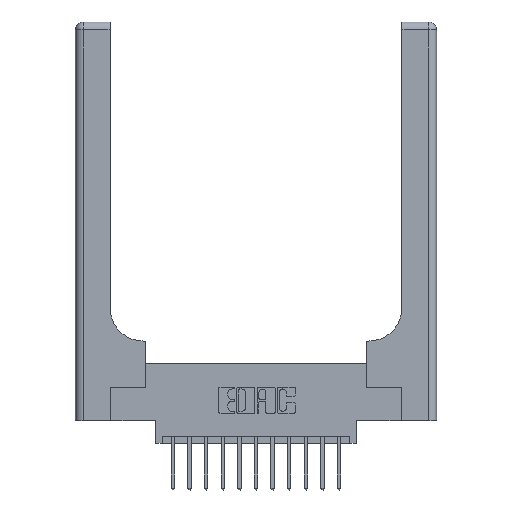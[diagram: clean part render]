
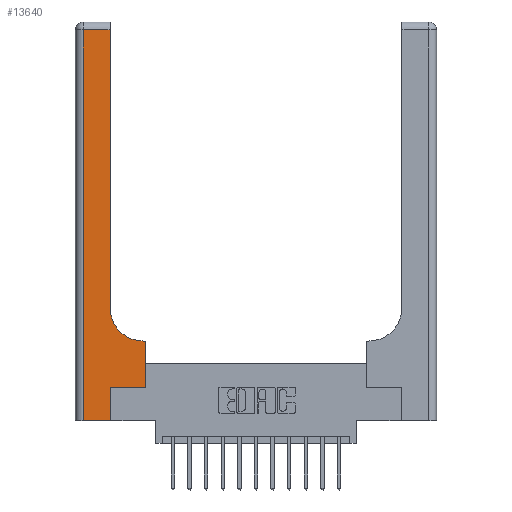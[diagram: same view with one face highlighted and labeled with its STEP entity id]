
A CAD part, top view. The second image highlights one B-rep face of the part: STEP entity #13640.
In plain terms, the highlighted planar face has unit normal (0, 0, 1).
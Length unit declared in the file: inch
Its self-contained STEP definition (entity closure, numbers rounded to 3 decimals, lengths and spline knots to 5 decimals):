
#272 = CARTESIAN_POINT ( 'NONE',  ( 0.265, 0.25, 0.37 ) ) ;
#301 = VECTOR ( 'NONE', #4578, 39.37008 ) ;
#364 = DIRECTION ( 'NONE',  ( 0., 1., 0. ) ) ;
#718 = CARTESIAN_POINT ( 'NONE',  ( 0., 0., 0.37 ) ) ;
#1066 = VECTOR ( 'NONE', #2626, 39.37008 ) ;
#1144 = CARTESIAN_POINT ( 'NONE',  ( 0.265, 0.25, 0.37 ) ) ;
#1217 = DIRECTION ( 'NONE',  ( 1., 0., 0. ) ) ;
#1365 = DIRECTION ( 'NONE',  ( 0., 0., -1. ) ) ;
#1498 = LINE ( 'NONE', #3154, #15614 ) ;
#1693 = EDGE_CURVE ( 'NONE', #6602, #12836, #7559, .T. ) ;
#1719 = CARTESIAN_POINT ( 'NONE',  ( 0., 2.94, 0.37 ) ) ;
#1975 = VERTEX_POINT ( 'NONE', #7046 ) ;
#2366 = EDGE_CURVE ( 'NONE', #8411, #1975, #9901, .T. ) ;
#2603 = ORIENTED_EDGE ( 'NONE', *, *, #16585, .T. ) ;
#2626 = DIRECTION ( 'NONE',  ( -1., 0., 0. ) ) ;
#3154 = CARTESIAN_POINT ( 'NONE',  ( 0.26, 3., 0.37 ) ) ;
#3428 = ORIENTED_EDGE ( 'NONE', *, *, #12887, .T. ) ;
#4018 = VERTEX_POINT ( 'NONE', #6866 ) ;
#4449 = LINE ( 'NONE', #7739, #1066 ) ;
#4478 = EDGE_CURVE ( 'NONE', #4018, #6602, #14662, .T. ) ;
#4578 = DIRECTION ( 'NONE',  ( 1., 0., 0. ) ) ;
#4962 = CARTESIAN_POINT ( 'NONE',  ( 0.528, 0.6, 0.37 ) ) ;
#5374 = EDGE_CURVE ( 'NONE', #12836, #7989, #5957, .T. ) ;
#5444 = CARTESIAN_POINT ( 'NONE',  ( 0.51, 0.85, 0.37 ) ) ;
#5725 = VECTOR ( 'NONE', #9416, 39.37008 ) ;
#5957 = LINE ( 'NONE', #13205, #12016 ) ;
#6065 = DIRECTION ( 'NONE',  ( 0., 1., 0. ) ) ;
#6602 = VERTEX_POINT ( 'NONE', #272 ) ;
#6757 = DIRECTION ( 'NONE',  ( 1., 0., 0. ) ) ;
#6866 = CARTESIAN_POINT ( 'NONE',  ( 0.265, 0., 0.37 ) ) ;
#7046 = CARTESIAN_POINT ( 'NONE',  ( 0.26, 0.85, 0.37 ) ) ;
#7147 = LINE ( 'NONE', #718, #301 ) ;
#7559 = LINE ( 'NONE', #1144, #10982 ) ;
#7636 = EDGE_CURVE ( 'NONE', #11572, #14128, #11759, .T. ) ;
#7713 = AXIS2_PLACEMENT_3D ( 'NONE', #9073, #1365, #10384 ) ;
#7739 = CARTESIAN_POINT ( 'NONE',  ( 0.26, 0.6, 0.37 ) ) ;
#7812 = VECTOR ( 'NONE', #6065, 39.37008 ) ;
#7989 = VERTEX_POINT ( 'NONE', #4962 ) ;
#8200 = CARTESIAN_POINT ( 'NONE',  ( 0.26, 2.94, 0.37 ) ) ;
#8296 = AXIS2_PLACEMENT_3D ( 'NONE', #5444, #14469, #6757 ) ;
#8310 = VECTOR ( 'NONE', #11907, 39.37008 ) ;
#8411 = VERTEX_POINT ( 'NONE', #8564 ) ;
#8476 = ORIENTED_EDGE ( 'NONE', *, *, #4478, .T. ) ;
#8564 = CARTESIAN_POINT ( 'NONE',  ( 0.51, 0.6, 0.37 ) ) ;
#8586 = ORIENTED_EDGE ( 'NONE', *, *, #7636, .T. ) ;
#8614 = CARTESIAN_POINT ( 'NONE',  ( 0.265, 0., 0.37 ) ) ;
#9073 = CARTESIAN_POINT ( 'NONE',  ( 0., 3., 0.37 ) ) ;
#9416 = DIRECTION ( 'NONE',  ( -1., 0., 0. ) ) ;
#9901 = CIRCLE ( 'NONE', #8296, 0.25 ) ;
#10336 = PLANE ( 'NONE',  #7713 ) ;
#10384 = DIRECTION ( 'NONE',  ( -1., 0., 0. ) ) ;
#10615 = CARTESIAN_POINT ( 'NONE',  ( 0.06, 3., 0.37 ) ) ;
#10982 = VECTOR ( 'NONE', #1217, 39.37008 ) ;
#11483 = VERTEX_POINT ( 'NONE', #8200 ) ;
#11572 = VERTEX_POINT ( 'NONE', #15028 ) ;
#11587 = EDGE_LOOP ( 'NONE', ( #2603, #16291, #8586, #3428, #8476, #13441, #15193, #12345, #12212 ) ) ;
#11759 = LINE ( 'NONE', #10615, #8310 ) ;
#11907 = DIRECTION ( 'NONE',  ( 0., -1., 0. ) ) ;
#12016 = VECTOR ( 'NONE', #364, 39.37008 ) ;
#12049 = EDGE_CURVE ( 'NONE', #11483, #11572, #15628, .T. ) ;
#12169 = DIRECTION ( 'NONE',  ( 0., 1., 0. ) ) ;
#12212 = ORIENTED_EDGE ( 'NONE', *, *, #2366, .T. ) ;
#12345 = ORIENTED_EDGE ( 'NONE', *, *, #14815, .T. ) ;
#12746 = CARTESIAN_POINT ( 'NONE',  ( 0.06, 0., 0.37 ) ) ;
#12836 = VERTEX_POINT ( 'NONE', #13487 ) ;
#12887 = EDGE_CURVE ( 'NONE', #14128, #4018, #7147, .T. ) ;
#12986 = FACE_OUTER_BOUND ( 'NONE', #11587, .T. ) ;
#13205 = CARTESIAN_POINT ( 'NONE',  ( 0.528, 0.25, 0.37 ) ) ;
#13441 = ORIENTED_EDGE ( 'NONE', *, *, #1693, .T. ) ;
#13487 = CARTESIAN_POINT ( 'NONE',  ( 0.528, 0.25, 0.37 ) ) ;
#13640 = ADVANCED_FACE ( 'NONE', ( #12986 ), #10336, .F. ) ;
#14128 = VERTEX_POINT ( 'NONE', #12746 ) ;
#14469 = DIRECTION ( 'NONE',  ( 0., 0., -1. ) ) ;
#14662 = LINE ( 'NONE', #8614, #7812 ) ;
#14815 = EDGE_CURVE ( 'NONE', #7989, #8411, #4449, .T. ) ;
#15028 = CARTESIAN_POINT ( 'NONE',  ( 0.06, 2.94, 0.37 ) ) ;
#15193 = ORIENTED_EDGE ( 'NONE', *, *, #5374, .T. ) ;
#15614 = VECTOR ( 'NONE', #12169, 39.37008 ) ;
#15628 = LINE ( 'NONE', #1719, #5725 ) ;
#16291 = ORIENTED_EDGE ( 'NONE', *, *, #12049, .T. ) ;
#16585 = EDGE_CURVE ( 'NONE', #1975, #11483, #1498, .T. ) ;
